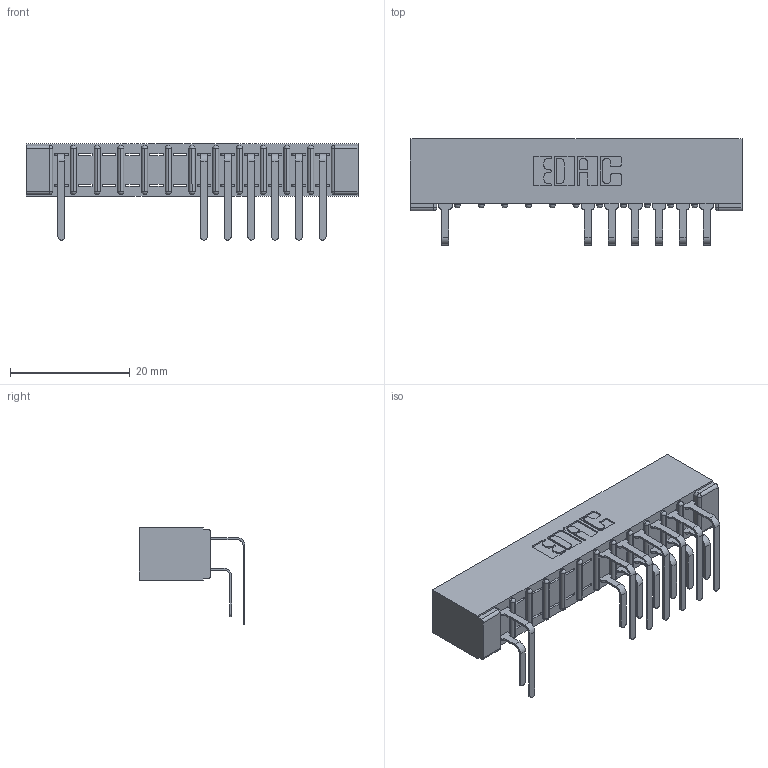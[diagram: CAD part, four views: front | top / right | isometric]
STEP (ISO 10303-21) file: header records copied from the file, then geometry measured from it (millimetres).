
FILE_DESCRIPTION (( 'STEP AP203' ), '1' );
FILE_NAME ('307-012-559-101.STEP', '2018-08-02T22:33:44', ( '' ), ( '' ), 'SwSTEP 2.0', 'SolidWorks 2016', '' );
FILE_SCHEMA (( 'CONFIG_CONTROL_DESIGN' ));
Length unit declared in the file: inch
Products named in the file (4): 307 Part_No Mounting Lugs; 307-290-001_558 559 - 1 (Single); 307-290-001_559 - 2 (Single); 307-012-559-101
Assembly tree (15 placements, depth 2):
  307-012-559-101
    307 Part_No Mounting Lugs
    307-290-001_558 559 - 1 (Single)  x7
    307-290-001_559 - 2 (Single)  x7
Bounding box: 55.42 x 17.69 x 16.08 mm (x, y, z)
Volume: 3792.1 mm3; surface area: 6231.7 mm2
Topology: 15 solids, 15 shells, 923 faces, 2607 edges, 1682 vertices
Faces by surface type: plane 588, cylinder 309, sphere 26
Entity records: 15219 total; most frequent: CARTESIAN_POINT 2540, ORIENTED_EDGE 2522, DIRECTION 2489, EDGE_CURVE 1261, LINE 955, VECTOR 955, VERTEX_POINT 818, AXIS2_PLACEMENT_3D 767
